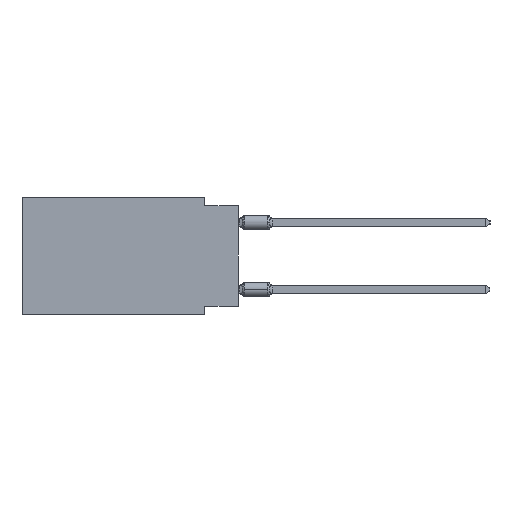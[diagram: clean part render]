
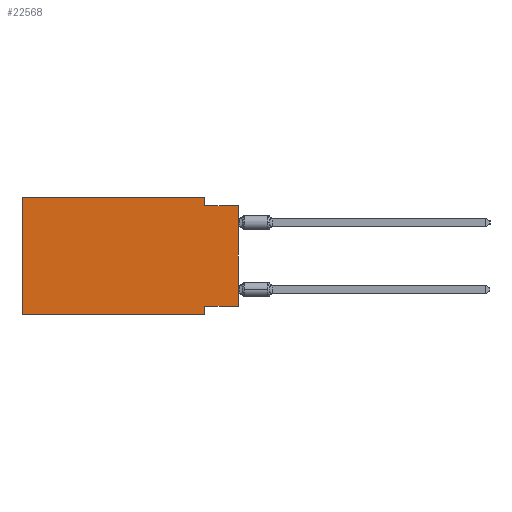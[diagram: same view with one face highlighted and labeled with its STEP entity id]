
A CAD part, left-side view. The second image highlights one B-rep face of the part: STEP entity #22568.
In plain terms, the highlighted planar face has unit normal (-1, 0, 0).
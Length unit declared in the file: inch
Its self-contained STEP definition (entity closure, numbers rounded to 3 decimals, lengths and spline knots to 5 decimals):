
#211 = VERTEX_POINT ( 'NONE', #686 ) ;
#568 = CARTESIAN_POINT ( 'NONE',  ( 0., 0.1, -0.025 ) ) ;
#686 = CARTESIAN_POINT ( 'NONE',  ( 0., 0.1, -0.35 ) ) ;
#937 = CARTESIAN_POINT ( 'NONE',  ( 0., 0.1, -0.325 ) ) ;
#1112 = EDGE_CURVE ( 'NONE', #59130, #211, #5180, .T. ) ;
#1520 = DIRECTION ( 'NONE',  ( 0., 0., -1. ) ) ;
#1599 = EDGE_CURVE ( 'NONE', #59130, #30196, #54192, .T. ) ;
#4344 = ORIENTED_EDGE ( 'NONE', *, *, #34299, .F. ) ;
#5180 = LINE ( 'NONE', #37246, #52109 ) ;
#7698 = VERTEX_POINT ( 'NONE', #47400 ) ;
#9560 = CARTESIAN_POINT ( 'NONE',  ( 0., 0.645, 0. ) ) ;
#10782 = DIRECTION ( 'NONE',  ( 1., 0., 0. ) ) ;
#11765 = VECTOR ( 'NONE', #59136, 39.37008 ) ;
#12201 = ORIENTED_EDGE ( 'NONE', *, *, #37439, .F. ) ;
#12243 = EDGE_LOOP ( 'NONE', ( #54383, #38147, #4344, #12201, #21121, #49223, #12459, #46415 ) ) ;
#12459 = ORIENTED_EDGE ( 'NONE', *, *, #58413, .F. ) ;
#17362 = CARTESIAN_POINT ( 'NONE',  ( 0., 0.1, 0. ) ) ;
#17511 = LINE ( 'NONE', #46843, #27939 ) ;
#18449 = VECTOR ( 'NONE', #47766, 39.37008 ) ;
#19253 = VECTOR ( 'NONE', #42706, 39.37008 ) ;
#20517 = EDGE_CURVE ( 'NONE', #22210, #33514, #38331, .T. ) ;
#20561 = CARTESIAN_POINT ( 'NONE',  ( 0., 0.645, 0. ) ) ;
#20748 = VECTOR ( 'NONE', #34800, 39.37008 ) ;
#21121 = ORIENTED_EDGE ( 'NONE', *, *, #1599, .F. ) ;
#21990 = DIRECTION ( 'NONE',  ( 0., 0., -1. ) ) ;
#22210 = VERTEX_POINT ( 'NONE', #31615 ) ;
#22292 = EDGE_CURVE ( 'NONE', #29425, #33514, #52580, .T. ) ;
#22568 = ADVANCED_FACE ( 'NONE', ( #37607 ), #56473, .F. ) ;
#24000 = DIRECTION ( 'NONE',  ( 0., -1., 0. ) ) ;
#25547 = VERTEX_POINT ( 'NONE', #937 ) ;
#26676 = VECTOR ( 'NONE', #21990, 39.37008 ) ;
#27939 = VECTOR ( 'NONE', #56421, 39.37008 ) ;
#28310 = LINE ( 'NONE', #32934, #18449 ) ;
#29425 = VERTEX_POINT ( 'NONE', #568 ) ;
#30196 = VERTEX_POINT ( 'NONE', #20561 ) ;
#31280 = CARTESIAN_POINT ( 'NONE',  ( 0., 0.645, -0.35 ) ) ;
#31615 = CARTESIAN_POINT ( 'NONE',  ( 0., 0., -0.325 ) ) ;
#32934 = CARTESIAN_POINT ( 'NONE',  ( 0., 0.1, -0.35 ) ) ;
#33433 = CARTESIAN_POINT ( 'NONE',  ( 0., 0., -0.025 ) ) ;
#33514 = VERTEX_POINT ( 'NONE', #60554 ) ;
#34299 = EDGE_CURVE ( 'NONE', #7698, #29425, #50093, .T. ) ;
#34800 = DIRECTION ( 'NONE',  ( 0., 1., 0. ) ) ;
#36804 = VECTOR ( 'NONE', #39248, 39.37008 ) ;
#37246 = CARTESIAN_POINT ( 'NONE',  ( 0., 0.645, -0.35 ) ) ;
#37439 = EDGE_CURVE ( 'NONE', #30196, #7698, #17511, .T. ) ;
#37607 = FACE_OUTER_BOUND ( 'NONE', #12243, .T. ) ;
#38147 = ORIENTED_EDGE ( 'NONE', *, *, #22292, .F. ) ;
#38331 = LINE ( 'NONE', #43582, #36804 ) ;
#39248 = DIRECTION ( 'NONE',  ( 0., 0., 1. ) ) ;
#40060 = LINE ( 'NONE', #48418, #20748 ) ;
#40295 = CARTESIAN_POINT ( 'NONE',  ( 0., 0.645, 0. ) ) ;
#42280 = EDGE_CURVE ( 'NONE', #22210, #25547, #40060, .T. ) ;
#42706 = DIRECTION ( 'NONE',  ( 0., -1., 0. ) ) ;
#43582 = CARTESIAN_POINT ( 'NONE',  ( 0., 0., 0. ) ) ;
#45906 = AXIS2_PLACEMENT_3D ( 'NONE', #9560, #10782, #1520 ) ;
#46415 = ORIENTED_EDGE ( 'NONE', *, *, #42280, .F. ) ;
#46843 = CARTESIAN_POINT ( 'NONE',  ( 0., 0.645, 0. ) ) ;
#47400 = CARTESIAN_POINT ( 'NONE',  ( 0., 0.1, 0. ) ) ;
#47766 = DIRECTION ( 'NONE',  ( 0., 0., -1. ) ) ;
#48418 = CARTESIAN_POINT ( 'NONE',  ( 0., 0., -0.325 ) ) ;
#49223 = ORIENTED_EDGE ( 'NONE', *, *, #1112, .T. ) ;
#50093 = LINE ( 'NONE', #17362, #26676 ) ;
#52109 = VECTOR ( 'NONE', #24000, 39.37008 ) ;
#52580 = LINE ( 'NONE', #33433, #19253 ) ;
#54192 = LINE ( 'NONE', #40295, #11765 ) ;
#54383 = ORIENTED_EDGE ( 'NONE', *, *, #20517, .T. ) ;
#56421 = DIRECTION ( 'NONE',  ( 0., -1., 0. ) ) ;
#56473 = PLANE ( 'NONE',  #45906 ) ;
#58413 = EDGE_CURVE ( 'NONE', #25547, #211, #28310, .T. ) ;
#59130 = VERTEX_POINT ( 'NONE', #31280 ) ;
#59136 = DIRECTION ( 'NONE',  ( 0., 0., 1. ) ) ;
#60554 = CARTESIAN_POINT ( 'NONE',  ( 0., 0., -0.025 ) ) ;
